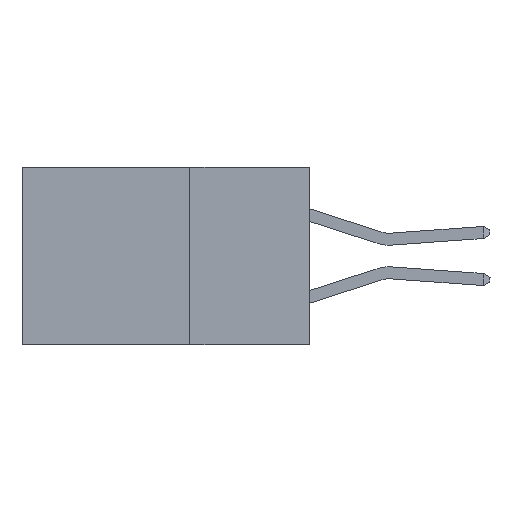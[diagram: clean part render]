
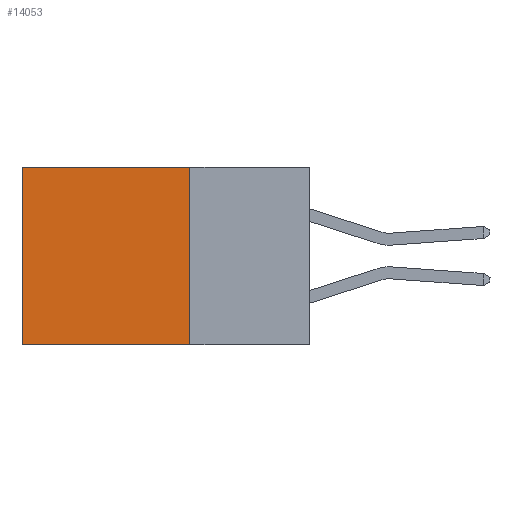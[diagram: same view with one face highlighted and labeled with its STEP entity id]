
A CAD part, left-side view. The second image highlights one B-rep face of the part: STEP entity #14053.
In plain terms, the highlighted planar face has unit normal (-1, 0, 0).
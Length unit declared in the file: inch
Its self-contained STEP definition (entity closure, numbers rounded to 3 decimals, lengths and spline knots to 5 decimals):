
#838 = CARTESIAN_POINT ( 'NONE',  ( 0.298, 0.6, 0. ) ) ;
#1002 = LINE ( 'NONE', #14514, #15342 ) ;
#1459 = VERTEX_POINT ( 'NONE', #16667 ) ;
#1997 = DIRECTION ( 'NONE',  ( 0., 1., 0. ) ) ;
#2242 = PLANE ( 'NONE',  #12513 ) ;
#2415 = CARTESIAN_POINT ( 'NONE',  ( 0.298, 0.25, 0. ) ) ;
#3324 = VERTEX_POINT ( 'NONE', #14420 ) ;
#3612 = CARTESIAN_POINT ( 'NONE',  ( 0.298, 0.25, -0.37 ) ) ;
#3683 = DIRECTION ( 'NONE',  ( 1., 0., 0. ) ) ;
#4319 = EDGE_CURVE ( 'NONE', #7812, #3324, #14352, .T. ) ;
#4669 = ORIENTED_EDGE ( 'NONE', *, *, #7454, .F. ) ;
#4718 = EDGE_CURVE ( 'NONE', #7750, #1459, #11109, .T. ) ;
#5290 = FACE_OUTER_BOUND ( 'NONE', #13382, .T. ) ;
#7342 = VECTOR ( 'NONE', #8851, 39.37008 ) ;
#7454 = EDGE_CURVE ( 'NONE', #1459, #3324, #17599, .T. ) ;
#7750 = VERTEX_POINT ( 'NONE', #2415 ) ;
#7812 = VERTEX_POINT ( 'NONE', #838 ) ;
#8670 = ORIENTED_EDGE ( 'NONE', *, *, #4718, .F. ) ;
#8851 = DIRECTION ( 'NONE',  ( 0., 0., -1. ) ) ;
#9587 = VECTOR ( 'NONE', #14545, 39.37008 ) ;
#11109 = LINE ( 'NONE', #13815, #7342 ) ;
#12304 = CARTESIAN_POINT ( 'NONE',  ( 0.298, 0.6, 0. ) ) ;
#12513 = AXIS2_PLACEMENT_3D ( 'NONE', #17310, #3683, #13398 ) ;
#12904 = ORIENTED_EDGE ( 'NONE', *, *, #16214, .T. ) ;
#13382 = EDGE_LOOP ( 'NONE', ( #17201, #4669, #8670, #12904 ) ) ;
#13398 = DIRECTION ( 'NONE',  ( 0., 0., -1. ) ) ;
#13629 = DIRECTION ( 'NONE',  ( 0., 0., -1. ) ) ;
#13815 = CARTESIAN_POINT ( 'NONE',  ( 0.298, 0.25, 0. ) ) ;
#14053 = ADVANCED_FACE ( 'NONE', ( #5290 ), #2242, .F. ) ;
#14352 = LINE ( 'NONE', #12304, #15159 ) ;
#14420 = CARTESIAN_POINT ( 'NONE',  ( 0.298, 0.6, -0.37 ) ) ;
#14514 = CARTESIAN_POINT ( 'NONE',  ( 0.298, 0.25, 0. ) ) ;
#14545 = DIRECTION ( 'NONE',  ( 0., 1., 0. ) ) ;
#15159 = VECTOR ( 'NONE', #13629, 39.37008 ) ;
#15342 = VECTOR ( 'NONE', #1997, 39.37008 ) ;
#16214 = EDGE_CURVE ( 'NONE', #7750, #7812, #1002, .T. ) ;
#16667 = CARTESIAN_POINT ( 'NONE',  ( 0.298, 0.25, -0.37 ) ) ;
#17201 = ORIENTED_EDGE ( 'NONE', *, *, #4319, .T. ) ;
#17310 = CARTESIAN_POINT ( 'NONE',  ( 0.298, 0.25, 0. ) ) ;
#17599 = LINE ( 'NONE', #3612, #9587 ) ;
